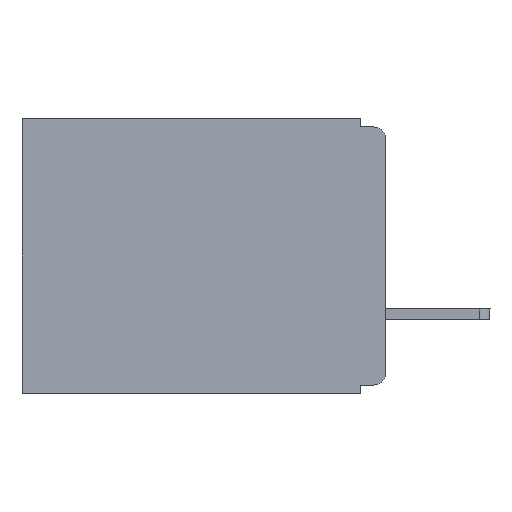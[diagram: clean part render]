
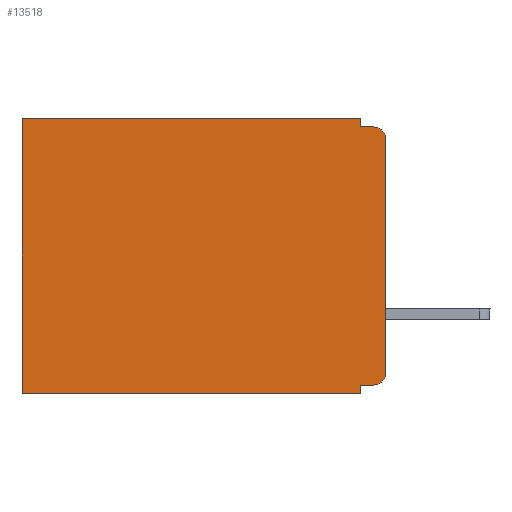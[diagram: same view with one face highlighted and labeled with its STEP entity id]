
A CAD part, left-side view. The second image highlights one B-rep face of the part: STEP entity #13518.
In plain terms, the highlighted planar face has unit normal (-1, 0, 0).
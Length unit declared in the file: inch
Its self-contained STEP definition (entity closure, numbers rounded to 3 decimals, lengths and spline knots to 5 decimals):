
#31 = ORIENTED_EDGE ( 'NONE', *, *, #6701, .F. ) ;
#567 = LINE ( 'NONE', #1593, #6211 ) ;
#650 = ORIENTED_EDGE ( 'NONE', *, *, #1452, .F. ) ;
#697 = FACE_OUTER_BOUND ( 'NONE', #3010, .T. ) ;
#875 = CARTESIAN_POINT ( 'NONE',  ( 0.3, 0.031, -0.01 ) ) ;
#890 = VECTOR ( 'NONE', #14719, 39.37008 ) ;
#904 = VECTOR ( 'NONE', #8409, 39.37008 ) ;
#978 = CARTESIAN_POINT ( 'NONE',  ( 0.3, 0.015, -0.01 ) ) ;
#1156 = LINE ( 'NONE', #13498, #3305 ) ;
#1452 = EDGE_CURVE ( 'NONE', #14279, #3160, #7762, .T. ) ;
#1593 = CARTESIAN_POINT ( 'NONE',  ( 0.3, 0., -0.01 ) ) ;
#1671 = EDGE_CURVE ( 'NONE', #5793, #5967, #5312, .T. ) ;
#1739 = EDGE_CURVE ( 'NONE', #3836, #14279, #11687, .T. ) ;
#1885 = CARTESIAN_POINT ( 'NONE',  ( 0.3, 0.031, -0.33 ) ) ;
#2195 = DIRECTION ( 'NONE',  ( -1., 0., 0. ) ) ;
#2254 = VERTEX_POINT ( 'NONE', #5703 ) ;
#2671 = VECTOR ( 'NONE', #5759, 39.37008 ) ;
#2843 = ORIENTED_EDGE ( 'NONE', *, *, #8797, .T. ) ;
#3010 = EDGE_LOOP ( 'NONE', ( #3380, #4445, #4331, #6140, #7513, #8412, #31, #650, #10335, #2843 ) ) ;
#3160 = VERTEX_POINT ( 'NONE', #6138 ) ;
#3286 = AXIS2_PLACEMENT_3D ( 'NONE', #6021, #9612, #11739 ) ;
#3305 = VECTOR ( 'NONE', #4330, 39.37008 ) ;
#3340 = DIRECTION ( 'NONE',  ( 1., 0., 0. ) ) ;
#3380 = ORIENTED_EDGE ( 'NONE', *, *, #1671, .F. ) ;
#3836 = VERTEX_POINT ( 'NONE', #9922 ) ;
#4330 = DIRECTION ( 'NONE',  ( 0., 0., -1. ) ) ;
#4331 = ORIENTED_EDGE ( 'NONE', *, *, #5661, .F. ) ;
#4359 = VERTEX_POINT ( 'NONE', #8952 ) ;
#4381 = VERTEX_POINT ( 'NONE', #10144 ) ;
#4445 = ORIENTED_EDGE ( 'NONE', *, *, #10767, .T. ) ;
#4529 = EDGE_CURVE ( 'NONE', #4359, #2254, #8019, .T. ) ;
#5312 = LINE ( 'NONE', #6744, #890 ) ;
#5661 = EDGE_CURVE ( 'NONE', #12899, #9407, #567, .T. ) ;
#5703 = CARTESIAN_POINT ( 'NONE',  ( 0.3, 0.437, -0.33 ) ) ;
#5727 = VECTOR ( 'NONE', #12607, 39.37008 ) ;
#5759 = DIRECTION ( 'NONE',  ( 0., 1., 0. ) ) ;
#5793 = VERTEX_POINT ( 'NONE', #14478 ) ;
#5967 = VERTEX_POINT ( 'NONE', #7992 ) ;
#5982 = CARTESIAN_POINT ( 'NONE',  ( 0.3, 0., -0.33 ) ) ;
#6021 = CARTESIAN_POINT ( 'NONE',  ( 0.3, 0.015, -0.305 ) ) ;
#6138 = CARTESIAN_POINT ( 'NONE',  ( 0.3, 0.031, -0.33 ) ) ;
#6140 = ORIENTED_EDGE ( 'NONE', *, *, #11682, .F. ) ;
#6211 = VECTOR ( 'NONE', #10652, 39.37008 ) ;
#6666 = DIRECTION ( 'NONE',  ( 0., 0., -1. ) ) ;
#6677 = DIRECTION ( 'NONE',  ( 0., 0., -1. ) ) ;
#6701 = EDGE_CURVE ( 'NONE', #3160, #2254, #6914, .T. ) ;
#6744 = CARTESIAN_POINT ( 'NONE',  ( 0.3, 0., -0.33 ) ) ;
#6847 = CARTESIAN_POINT ( 'NONE',  ( 0.3, 0., -0.32 ) ) ;
#6914 = LINE ( 'NONE', #5982, #904 ) ;
#7245 = VECTOR ( 'NONE', #7598, 39.37008 ) ;
#7418 = PLANE ( 'NONE',  #9384 ) ;
#7513 = ORIENTED_EDGE ( 'NONE', *, *, #12929, .T. ) ;
#7598 = DIRECTION ( 'NONE',  ( 0., 0., -1. ) ) ;
#7762 = LINE ( 'NONE', #1885, #7245 ) ;
#7992 = CARTESIAN_POINT ( 'NONE',  ( 0.3, 0., -0.305 ) ) ;
#8019 = LINE ( 'NONE', #10328, #5727 ) ;
#8409 = DIRECTION ( 'NONE',  ( 0., 1., 0. ) ) ;
#8412 = ORIENTED_EDGE ( 'NONE', *, *, #4529, .T. ) ;
#8545 = LINE ( 'NONE', #13313, #14594 ) ;
#8797 = EDGE_CURVE ( 'NONE', #3836, #5967, #10120, .T. ) ;
#8952 = CARTESIAN_POINT ( 'NONE',  ( 0.3, 0.437, 0. ) ) ;
#9384 = AXIS2_PLACEMENT_3D ( 'NONE', #12222, #3340, #6666 ) ;
#9407 = VERTEX_POINT ( 'NONE', #978 ) ;
#9612 = DIRECTION ( 'NONE',  ( -1., 0., 0. ) ) ;
#9922 = CARTESIAN_POINT ( 'NONE',  ( 0.3, 0.015, -0.32 ) ) ;
#10120 = CIRCLE ( 'NONE', #3286, 0.015 ) ;
#10144 = CARTESIAN_POINT ( 'NONE',  ( 0.3, 0.031, 0. ) ) ;
#10328 = CARTESIAN_POINT ( 'NONE',  ( 0.3, 0.437, -0.33 ) ) ;
#10335 = ORIENTED_EDGE ( 'NONE', *, *, #1739, .F. ) ;
#10652 = DIRECTION ( 'NONE',  ( 0., -1., 0. ) ) ;
#10763 = CARTESIAN_POINT ( 'NONE',  ( 0.3, 0.015, -0.025 ) ) ;
#10767 = EDGE_CURVE ( 'NONE', #5793, #9407, #12163, .T. ) ;
#11682 = EDGE_CURVE ( 'NONE', #4381, #12899, #1156, .T. ) ;
#11687 = LINE ( 'NONE', #6847, #2671 ) ;
#11739 = DIRECTION ( 'NONE',  ( 0., 0., -1. ) ) ;
#12163 = CIRCLE ( 'NONE', #14223, 0.015 ) ;
#12222 = CARTESIAN_POINT ( 'NONE',  ( 0.3, 0., -0.33 ) ) ;
#12607 = DIRECTION ( 'NONE',  ( 0., 0., -1. ) ) ;
#12899 = VERTEX_POINT ( 'NONE', #875 ) ;
#12929 = EDGE_CURVE ( 'NONE', #4381, #4359, #8545, .T. ) ;
#13313 = CARTESIAN_POINT ( 'NONE',  ( 0.3, 0., 0. ) ) ;
#13498 = CARTESIAN_POINT ( 'NONE',  ( 0.3, 0.031, 0. ) ) ;
#13518 = ADVANCED_FACE ( 'NONE', ( #697 ), #7418, .F. ) ;
#14178 = CARTESIAN_POINT ( 'NONE',  ( 0.3, 0.031, -0.32 ) ) ;
#14223 = AXIS2_PLACEMENT_3D ( 'NONE', #10763, #2195, #6677 ) ;
#14279 = VERTEX_POINT ( 'NONE', #14178 ) ;
#14451 = DIRECTION ( 'NONE',  ( 0., 1., 0. ) ) ;
#14478 = CARTESIAN_POINT ( 'NONE',  ( 0.3, 0., -0.025 ) ) ;
#14594 = VECTOR ( 'NONE', #14451, 39.37008 ) ;
#14719 = DIRECTION ( 'NONE',  ( 0., 0., -1. ) ) ;
